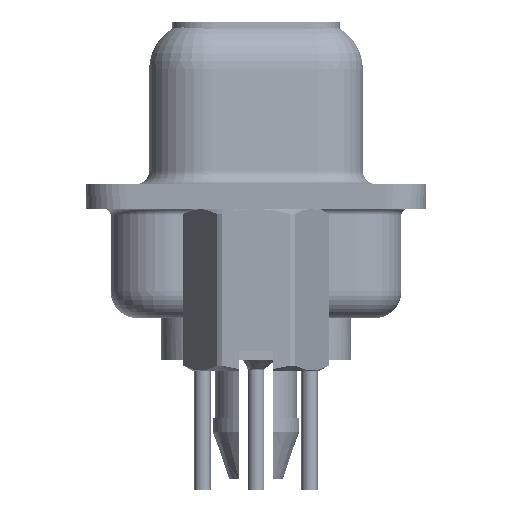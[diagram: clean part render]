
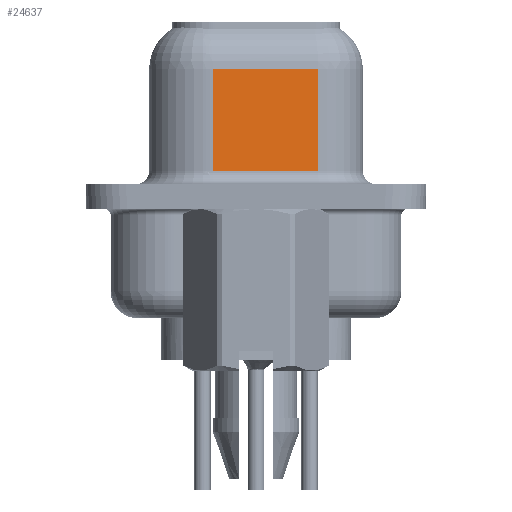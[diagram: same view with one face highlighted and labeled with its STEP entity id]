
A CAD part, left-side view. The second image highlights one B-rep face of the part: STEP entity #24637.
In plain terms, the highlighted planar face has unit normal (-0.985, -0.174, 0).
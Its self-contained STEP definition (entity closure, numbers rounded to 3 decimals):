
#93 = VECTOR ( 'NONE', #12277, 1000. ) ;
#1099 = ORIENTED_EDGE ( 'NONE', *, *, #28158, .T. ) ;
#1256 = CARTESIAN_POINT ( 'NONE',  ( 5.053, -2.297, 6.45 ) ) ;
#1911 = ORIENTED_EDGE ( 'NONE', *, *, #23815, .F. ) ;
#6768 = CARTESIAN_POINT ( 'NONE',  ( 4.365, 1.603, 6.45 ) ) ;
#7361 = CARTESIAN_POINT ( 'NONE',  ( 5.053, -2.297, 6.45 ) ) ;
#7462 = CARTESIAN_POINT ( 'NONE',  ( 5.053, -2.297, 4.7 ) ) ;
#10094 = CARTESIAN_POINT ( 'NONE',  ( 5.053, -2.297, 4.7 ) ) ;
#11814 = CARTESIAN_POINT ( 'NONE',  ( 5.053, -2.297, 0.95 ) ) ;
#12277 = DIRECTION ( 'NONE',  ( 0., 0., -1. ) ) ;
#12838 = VERTEX_POINT ( 'NONE', #33286 ) ;
#12880 = EDGE_LOOP ( 'NONE', ( #1911, #31330, #1099, #17844 ) ) ;
#15008 = LINE ( 'NONE', #6768, #93 ) ;
#17844 = ORIENTED_EDGE ( 'NONE', *, *, #23281, .T. ) ;
#17855 = DIRECTION ( 'NONE',  ( 0., 0., -1. ) ) ;
#19270 = FACE_OUTER_BOUND ( 'NONE', #12880, .T. ) ;
#19860 = EDGE_CURVE ( 'NONE', #33246, #32487, #33791, .T. ) ;
#20309 = LINE ( 'NONE', #22551, #23980 ) ;
#20588 = VECTOR ( 'NONE', #25680, 1000. ) ;
#21302 = LINE ( 'NONE', #7361, #33379 ) ;
#22023 = DIRECTION ( 'NONE',  ( -0.174, 0.985, 0. ) ) ;
#22551 = CARTESIAN_POINT ( 'NONE',  ( 5.053, -2.297, 0.95 ) ) ;
#23281 = EDGE_CURVE ( 'NONE', #12838, #25184, #20309, .T. ) ;
#23815 = EDGE_CURVE ( 'NONE', #33246, #25184, #21302, .T. ) ;
#23980 = VECTOR ( 'NONE', #33067, 1000. ) ;
#24637 = ADVANCED_FACE ( 'NONE', ( #19270 ), #24928, .F. ) ;
#24928 = PLANE ( 'NONE',  #27364 ) ;
#25184 = VERTEX_POINT ( 'NONE', #11814 ) ;
#25680 = DIRECTION ( 'NONE',  ( -0.174, 0.985, 0. ) ) ;
#25879 = CARTESIAN_POINT ( 'NONE',  ( 4.365, 1.603, 4.7 ) ) ;
#27157 = DIRECTION ( 'NONE',  ( 0.985, 0.174, 0. ) ) ;
#27364 = AXIS2_PLACEMENT_3D ( 'NONE', #1256, #27157, #22023 ) ;
#28158 = EDGE_CURVE ( 'NONE', #32487, #12838, #15008, .T. ) ;
#31330 = ORIENTED_EDGE ( 'NONE', *, *, #19860, .T. ) ;
#32487 = VERTEX_POINT ( 'NONE', #25879 ) ;
#33067 = DIRECTION ( 'NONE',  ( 0.174, -0.985, 0. ) ) ;
#33246 = VERTEX_POINT ( 'NONE', #10094 ) ;
#33286 = CARTESIAN_POINT ( 'NONE',  ( 4.365, 1.603, 0.95 ) ) ;
#33379 = VECTOR ( 'NONE', #17855, 1000. ) ;
#33791 = LINE ( 'NONE', #7462, #20588 ) ;
